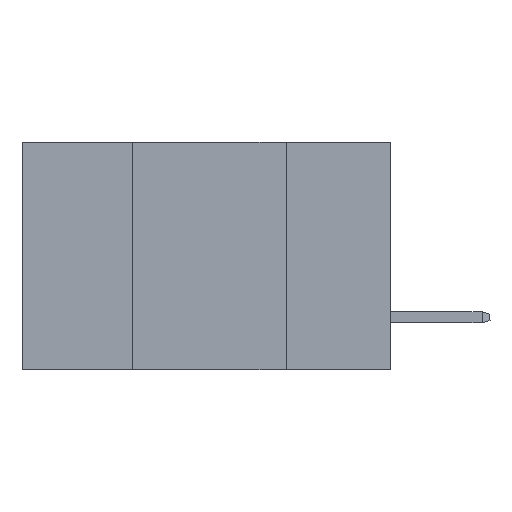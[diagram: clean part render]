
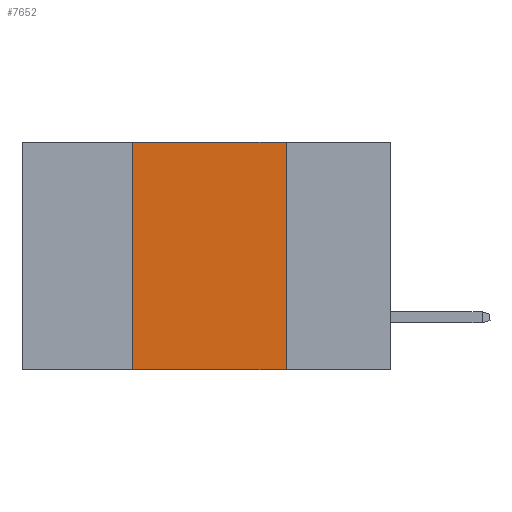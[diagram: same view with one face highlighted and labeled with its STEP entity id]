
A CAD part, left-side view. The second image highlights one B-rep face of the part: STEP entity #7652.
In plain terms, the highlighted planar face has unit normal (-1, 0, 0).
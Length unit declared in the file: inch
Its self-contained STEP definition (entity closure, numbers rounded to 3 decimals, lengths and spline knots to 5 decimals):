
#86 = ORIENTED_EDGE ( 'NONE', *, *, #12607, .F. ) ;
#1155 = VECTOR ( 'NONE', #10408, 39.37008 ) ;
#1661 = CARTESIAN_POINT ( 'NONE',  ( 0., 0.6, 0. ) ) ;
#2254 = CARTESIAN_POINT ( 'NONE',  ( 0., 0.42, 0. ) ) ;
#2278 = VERTEX_POINT ( 'NONE', #5506 ) ;
#2406 = CARTESIAN_POINT ( 'NONE',  ( 0., 0.17, 0. ) ) ;
#2753 = LINE ( 'NONE', #12450, #14887 ) ;
#3072 = VERTEX_POINT ( 'NONE', #2406 ) ;
#3349 = ORIENTED_EDGE ( 'NONE', *, *, #12825, .F. ) ;
#3775 = ORIENTED_EDGE ( 'NONE', *, *, #8145, .T. ) ;
#4129 = PLANE ( 'NONE',  #7002 ) ;
#4142 = DIRECTION ( 'NONE',  ( 0., 0., -1. ) ) ;
#4248 = EDGE_LOOP ( 'NONE', ( #86, #3349, #4817, #3775 ) ) ;
#4352 = CARTESIAN_POINT ( 'NONE',  ( 0., 0.17, -0.37 ) ) ;
#4817 = ORIENTED_EDGE ( 'NONE', *, *, #11106, .F. ) ;
#5338 = DIRECTION ( 'NONE',  ( 1., 0., 0. ) ) ;
#5506 = CARTESIAN_POINT ( 'NONE',  ( 0., 0.42, -0.37 ) ) ;
#5769 = LINE ( 'NONE', #12107, #8792 ) ;
#6531 = VERTEX_POINT ( 'NONE', #2254 ) ;
#6908 = DIRECTION ( 'NONE',  ( 0., -1., 0. ) ) ;
#7002 = AXIS2_PLACEMENT_3D ( 'NONE', #1661, #5338, #13246 ) ;
#7107 = DIRECTION ( 'NONE',  ( 0., 0., 1. ) ) ;
#7652 = ADVANCED_FACE ( 'NONE', ( #13518 ), #4129, .F. ) ;
#8145 = EDGE_CURVE ( 'NONE', #2278, #13705, #13502, .T. ) ;
#8792 = VECTOR ( 'NONE', #4142, 39.37008 ) ;
#9179 = LINE ( 'NONE', #13768, #11750 ) ;
#10408 = DIRECTION ( 'NONE',  ( 0., -1., 0. ) ) ;
#11106 = EDGE_CURVE ( 'NONE', #2278, #6531, #9179, .T. ) ;
#11750 = VECTOR ( 'NONE', #7107, 39.37008 ) ;
#12107 = CARTESIAN_POINT ( 'NONE',  ( 0., 0.17, 0. ) ) ;
#12450 = CARTESIAN_POINT ( 'NONE',  ( 0., 0.6, 0. ) ) ;
#12607 = EDGE_CURVE ( 'NONE', #3072, #13705, #5769, .T. ) ;
#12825 = EDGE_CURVE ( 'NONE', #6531, #3072, #2753, .T. ) ;
#13246 = DIRECTION ( 'NONE',  ( 0., 0., -1. ) ) ;
#13502 = LINE ( 'NONE', #15060, #1155 ) ;
#13518 = FACE_OUTER_BOUND ( 'NONE', #4248, .T. ) ;
#13705 = VERTEX_POINT ( 'NONE', #4352 ) ;
#13768 = CARTESIAN_POINT ( 'NONE',  ( 0., 0.42, 0. ) ) ;
#14887 = VECTOR ( 'NONE', #6908, 39.37008 ) ;
#15060 = CARTESIAN_POINT ( 'NONE',  ( 0., 0.6, -0.37 ) ) ;
